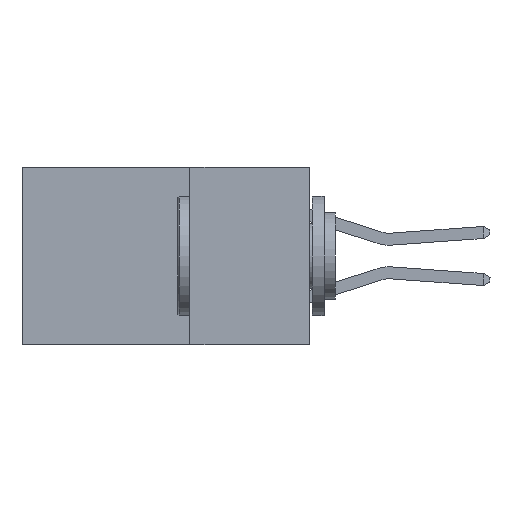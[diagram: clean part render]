
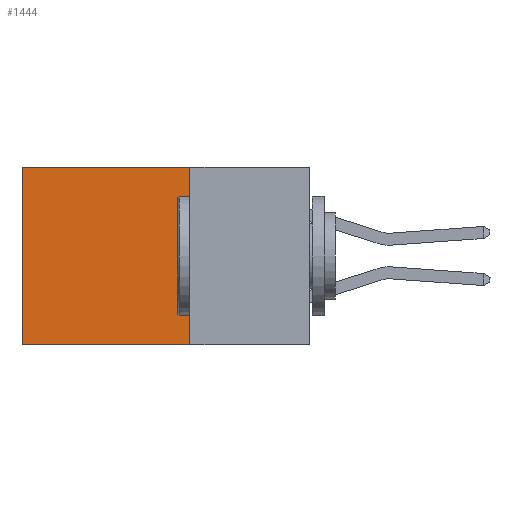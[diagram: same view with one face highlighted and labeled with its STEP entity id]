
A CAD part, left-side view. The second image highlights one B-rep face of the part: STEP entity #1444.
In plain terms, the highlighted planar face has unit normal (-1, 0, 0).
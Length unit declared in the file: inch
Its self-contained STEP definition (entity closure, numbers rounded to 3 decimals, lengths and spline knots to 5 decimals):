
#94 = FACE_OUTER_BOUND ( 'NONE', #12146, .T. ) ;
#383 = VECTOR ( 'NONE', #11680, 39.37008 ) ;
#456 = DIRECTION ( 'NONE',  ( 0., 0., -1. ) ) ;
#537 = DIRECTION ( 'NONE',  ( 0., 0., -1. ) ) ;
#1444 = ADVANCED_FACE ( 'NONE', ( #94 ), #9338, .F. ) ;
#2119 = ORIENTED_EDGE ( 'NONE', *, *, #9957, .F. ) ;
#2579 = CARTESIAN_POINT ( 'NONE',  ( 0.298, 0.6, 0. ) ) ;
#2745 = VERTEX_POINT ( 'NONE', #5893 ) ;
#4353 = LINE ( 'NONE', #14477, #383 ) ;
#5065 = DIRECTION ( 'NONE',  ( 0., 0., -1. ) ) ;
#5268 = ORIENTED_EDGE ( 'NONE', *, *, #18084, .T. ) ;
#5893 = CARTESIAN_POINT ( 'NONE',  ( 0.298, 0.6, -0.37 ) ) ;
#5965 = LINE ( 'NONE', #12275, #9389 ) ;
#6186 = ORIENTED_EDGE ( 'NONE', *, *, #17089, .T. ) ;
#7325 = EDGE_CURVE ( 'NONE', #13479, #2745, #12118, .T. ) ;
#8157 = LINE ( 'NONE', #10778, #15380 ) ;
#8512 = CARTESIAN_POINT ( 'NONE',  ( 0.298, 0.25, -0.37 ) ) ;
#9007 = VERTEX_POINT ( 'NONE', #16504 ) ;
#9338 = PLANE ( 'NONE',  #13344 ) ;
#9389 = VECTOR ( 'NONE', #5065, 39.37008 ) ;
#9616 = VERTEX_POINT ( 'NONE', #2579 ) ;
#9957 = EDGE_CURVE ( 'NONE', #9007, #13479, #8157, .T. ) ;
#10778 = CARTESIAN_POINT ( 'NONE',  ( 0.298, 0.25, 0. ) ) ;
#11555 = ORIENTED_EDGE ( 'NONE', *, *, #7325, .F. ) ;
#11667 = VECTOR ( 'NONE', #18410, 39.37008 ) ;
#11680 = DIRECTION ( 'NONE',  ( 0., 1., 0. ) ) ;
#12041 = CARTESIAN_POINT ( 'NONE',  ( 0.298, 0.25, 0. ) ) ;
#12118 = LINE ( 'NONE', #18380, #11667 ) ;
#12146 = EDGE_LOOP ( 'NONE', ( #6186, #11555, #2119, #5268 ) ) ;
#12275 = CARTESIAN_POINT ( 'NONE',  ( 0.298, 0.6, 0. ) ) ;
#13344 = AXIS2_PLACEMENT_3D ( 'NONE', #12041, #16718, #456 ) ;
#13479 = VERTEX_POINT ( 'NONE', #8512 ) ;
#14477 = CARTESIAN_POINT ( 'NONE',  ( 0.298, 0.25, 0. ) ) ;
#15380 = VECTOR ( 'NONE', #537, 39.37008 ) ;
#16504 = CARTESIAN_POINT ( 'NONE',  ( 0.298, 0.25, 0. ) ) ;
#16718 = DIRECTION ( 'NONE',  ( 1., 0., 0. ) ) ;
#17089 = EDGE_CURVE ( 'NONE', #9616, #2745, #5965, .T. ) ;
#18084 = EDGE_CURVE ( 'NONE', #9007, #9616, #4353, .T. ) ;
#18380 = CARTESIAN_POINT ( 'NONE',  ( 0.298, 0.25, -0.37 ) ) ;
#18410 = DIRECTION ( 'NONE',  ( 0., 1., 0. ) ) ;
